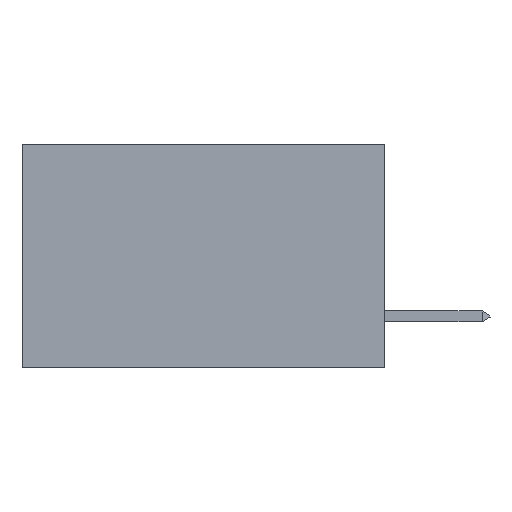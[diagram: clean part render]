
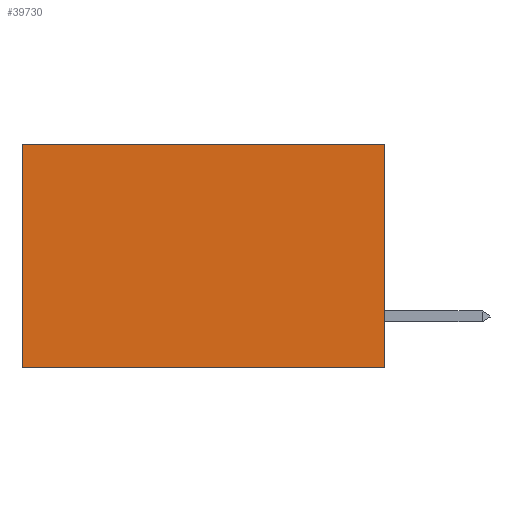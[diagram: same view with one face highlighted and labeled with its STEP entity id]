
A CAD part, left-side view. The second image highlights one B-rep face of the part: STEP entity #39730.
In plain terms, the highlighted planar face has unit normal (-1, 0, 0).
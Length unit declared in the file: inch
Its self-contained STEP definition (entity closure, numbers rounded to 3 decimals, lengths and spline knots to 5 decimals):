
#256 = VECTOR ( 'NONE', #35158, 39.37008 ) ;
#1192 = CARTESIAN_POINT ( 'NONE',  ( 0.2875, 0., 0. ) ) ;
#1929 = CARTESIAN_POINT ( 'NONE',  ( 0.2875, 0., 0. ) ) ;
#2654 = CARTESIAN_POINT ( 'NONE',  ( 0.2875, 0., -0.37 ) ) ;
#2664 = VERTEX_POINT ( 'NONE', #33859 ) ;
#5971 = EDGE_LOOP ( 'NONE', ( #44209, #27499, #29968, #22799 ) ) ;
#8257 = VECTOR ( 'NONE', #42045, 39.37008 ) ;
#10132 = EDGE_CURVE ( 'NONE', #2664, #11248, #10816, .T. ) ;
#10816 = LINE ( 'NONE', #1929, #256 ) ;
#11248 = VERTEX_POINT ( 'NONE', #35304 ) ;
#11290 = EDGE_CURVE ( 'NONE', #38846, #25189, #40370, .T. ) ;
#12828 = EDGE_CURVE ( 'NONE', #2664, #38846, #44883, .T. ) ;
#13188 = CARTESIAN_POINT ( 'NONE',  ( 0.2875, 0., -0.37 ) ) ;
#16776 = CARTESIAN_POINT ( 'NONE',  ( 0.2875, 0.6, -0.37 ) ) ;
#17414 = DIRECTION ( 'NONE',  ( 0., 1., 0. ) ) ;
#18280 = VECTOR ( 'NONE', #17414, 39.37008 ) ;
#22799 = ORIENTED_EDGE ( 'NONE', *, *, #10132, .T. ) ;
#25189 = VERTEX_POINT ( 'NONE', #16776 ) ;
#27499 = ORIENTED_EDGE ( 'NONE', *, *, #11290, .F. ) ;
#27621 = DIRECTION ( 'NONE',  ( 0., 0., -1. ) ) ;
#28965 = DIRECTION ( 'NONE',  ( 1., 0., 0. ) ) ;
#29968 = ORIENTED_EDGE ( 'NONE', *, *, #12828, .F. ) ;
#33235 = EDGE_CURVE ( 'NONE', #11248, #25189, #43511, .T. ) ;
#33859 = CARTESIAN_POINT ( 'NONE',  ( 0.2875, 0., 0. ) ) ;
#35158 = DIRECTION ( 'NONE',  ( 0., 1., 0. ) ) ;
#35304 = CARTESIAN_POINT ( 'NONE',  ( 0.2875, 0.6, 0. ) ) ;
#38846 = VERTEX_POINT ( 'NONE', #2654 ) ;
#39394 = FACE_OUTER_BOUND ( 'NONE', #5971, .T. ) ;
#39457 = VECTOR ( 'NONE', #27621, 39.37008 ) ;
#39730 = ADVANCED_FACE ( 'NONE', ( #39394 ), #47340, .F. ) ;
#40370 = LINE ( 'NONE', #13188, #18280 ) ;
#40496 = CARTESIAN_POINT ( 'NONE',  ( 0.2875, 0., 0. ) ) ;
#42045 = DIRECTION ( 'NONE',  ( 0., 0., -1. ) ) ;
#43511 = LINE ( 'NONE', #45956, #39457 ) ;
#43729 = DIRECTION ( 'NONE',  ( 0., 0., -1. ) ) ;
#44209 = ORIENTED_EDGE ( 'NONE', *, *, #33235, .T. ) ;
#44883 = LINE ( 'NONE', #1192, #8257 ) ;
#45723 = AXIS2_PLACEMENT_3D ( 'NONE', #40496, #28965, #43729 ) ;
#45956 = CARTESIAN_POINT ( 'NONE',  ( 0.2875, 0.6, 0. ) ) ;
#47340 = PLANE ( 'NONE',  #45723 ) ;
